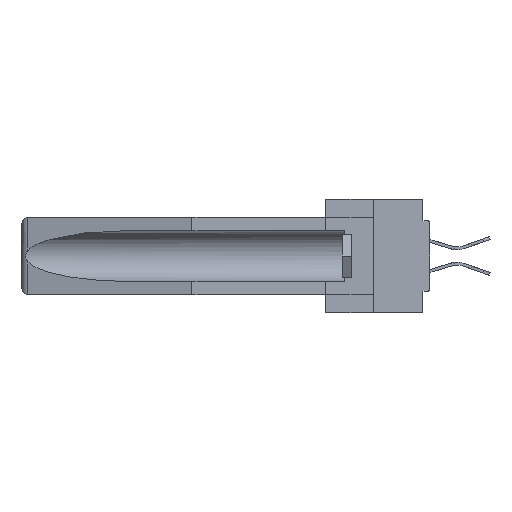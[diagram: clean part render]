
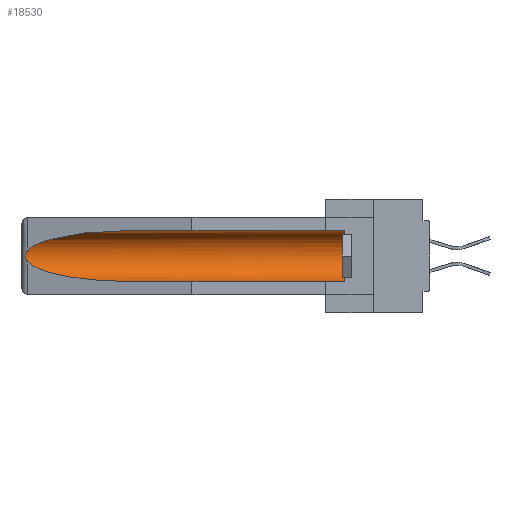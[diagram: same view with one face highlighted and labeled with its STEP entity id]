
A CAD part, left-side view. The second image highlights one B-rep face of the part: STEP entity #18530.
In plain terms, the highlighted cylindrical face has radius 2.857 mm (diameter 5.715 mm), a partial arc.
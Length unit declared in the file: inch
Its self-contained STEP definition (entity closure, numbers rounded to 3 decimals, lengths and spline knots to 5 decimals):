
#882 = AXIS2_PLACEMENT_3D ( 'NONE', #37598, #18203, #40894 ) ;
#1611 = CARTESIAN_POINT ( 'NONE',  ( 0.26537, 1.52718, -0.14972 ) ) ;
#3280 = CARTESIAN_POINT ( 'NONE',  ( 0.26597, 1.5296, -0.19026 ) ) ;
#3557 = CARTESIAN_POINT ( 'NONE',  ( 0.26537, 1.52718, -0.19328 ) ) ;
#3558 = VECTOR ( 'NONE', #12889, 39.37008 ) ;
#3922 = ORIENTED_EDGE ( 'NONE', *, *, #5199, .T. ) ;
#5050 = CARTESIAN_POINT ( 'NONE',  ( 0.155, -0.30754, -0.1715 ) ) ;
#5131 = ORIENTED_EDGE ( 'NONE', *, *, #38512, .T. ) ;
#5199 = EDGE_CURVE ( 'NONE', #19929, #33676, #34286, .T. ) ;
#6476 = CARTESIAN_POINT ( 'NONE',  ( 0.26597, 1.52961, -0.15275 ) ) ;
#9622 = EDGE_CURVE ( 'NONE', #16910, #29079, #25390, .T. ) ;
#9692 = CARTESIAN_POINT ( 'NONE',  ( 0.2673, 1.53269, -0.17917 ) ) ;
#10557 = EDGE_LOOP ( 'NONE', ( #22470, #5131, #3922, #35217, #26664, #25958 ) ) ;
#10657 = EDGE_CURVE ( 'NONE', #10664, #16910, #38029, .T. ) ;
#10664 = VERTEX_POINT ( 'NONE', #16553 ) ;
#11248 = VECTOR ( 'NONE', #35935, 39.37008 ) ;
#12256 = CARTESIAN_POINT ( 'NONE',  ( 0.25451, 1.48313, -0.24835 ) ) ;
#12609 = CARTESIAN_POINT ( 'NONE',  ( 0.2675, 1.53308, -0.16763 ) ) ;
#12748 = CARTESIAN_POINT ( 'NONE',  ( 0.155, -0.30754, -0.284 ) ) ;
#12889 = DIRECTION ( 'NONE',  ( 0., 1., 0. ) ) ;
#14210 = FACE_OUTER_BOUND ( 'NONE', #10557, .T. ) ;
#14325 = CARTESIAN_POINT ( 'NONE',  ( 0.26537, 1.52718, -0.19328 ) ) ;
#16044 = CARTESIAN_POINT ( 'NONE',  ( 0.155, 1.07973, -0.284 ) ) ;
#16129 = CARTESIAN_POINT ( 'NONE',  ( 0.2673, 1.5327, -0.16383 ) ) ;
#16184 = CARTESIAN_POINT ( 'NONE',  ( 0.21114, 1.30732, -0.284 ) ) ;
#16553 = CARTESIAN_POINT ( 'NONE',  ( 0.155, 0.126, -0.059 ) ) ;
#16910 = VERTEX_POINT ( 'NONE', #19436 ) ;
#18069 = DIRECTION ( 'NONE',  ( 0., 1., 0. ) ) ;
#18203 = DIRECTION ( 'NONE',  ( 0., -1., 0. ) ) ;
#18367 = CARTESIAN_POINT ( 'NONE',  ( 0.155, 1.07973, -0.284 ) ) ;
#18530 = ADVANCED_FACE ( 'NONE', ( #14210 ), #31381, .F. ) ;
#18571 = EDGE_CURVE ( 'NONE', #36575, #10664, #24782, .T. ) ;
#18821 = CARTESIAN_POINT ( 'NONE',  ( 0.26537, 1.52718, -0.19328 ) ) ;
#19436 = CARTESIAN_POINT ( 'NONE',  ( 0.155, 1.07973, -0.059 ) ) ;
#19929 = VERTEX_POINT ( 'NONE', #14325 ) ;
#21216 = CARTESIAN_POINT ( 'NONE',  ( 0.25451, 1.48313, -0.09465 ) ) ;
#21594 = LINE ( 'NONE', #12748, #3558 ) ;
#22470 = ORIENTED_EDGE ( 'NONE', *, *, #9622, .T. ) ;
#22479 = CARTESIAN_POINT ( 'NONE',  ( 0.26655, 1.53094, -0.18657 ) ) ;
#22613 = CARTESIAN_POINT ( 'NONE',  ( 0.155, -0.30754, -0.059 ) ) ;
#23965 = CARTESIAN_POINT ( 'NONE',  ( 0.155, 1.07973, -0.059 ) ) ;
#24782 = CIRCLE ( 'NONE', #882, 0.1125 ) ;
#25390 =( BOUNDED_CURVE ( )  B_SPLINE_CURVE ( 3, ( #23965, #30434, #21216, #36985 ),
 .UNSPECIFIED., .F., .F. ) 
 B_SPLINE_CURVE_WITH_KNOTS ( ( 4, 4 ),
 ( 4.71239, 6.08839 ),
 .UNSPECIFIED. ) 
 CURVE ( )  GEOMETRIC_REPRESENTATION_ITEM ( )  RATIONAL_B_SPLINE_CURVE ( ( 1., 0.848, 0.848, 1. ) ) 
 REPRESENTATION_ITEM ( '' )  );
#25958 = ORIENTED_EDGE ( 'NONE', *, *, #10657, .T. ) ;
#26664 = ORIENTED_EDGE ( 'NONE', *, *, #18571, .T. ) ;
#29079 = VERTEX_POINT ( 'NONE', #1611 ) ;
#29086 = CARTESIAN_POINT ( 'NONE',  ( 0.2675, 1.53308, -0.17534 ) ) ;
#29150 = CARTESIAN_POINT ( 'NONE',  ( 0.155, 0.126, -0.284 ) ) ;
#30434 = CARTESIAN_POINT ( 'NONE',  ( 0.21114, 1.30732, -0.059 ) ) ;
#31381 = CYLINDRICAL_SURFACE ( 'NONE', #35075, 0.1125 ) ;
#33676 = VERTEX_POINT ( 'NONE', #16044 ) ;
#34286 =( BOUNDED_CURVE ( )  B_SPLINE_CURVE ( 3, ( #18821, #12256, #16184, #18367 ),
 .UNSPECIFIED., .F., .F. ) 
 B_SPLINE_CURVE_WITH_KNOTS ( ( 4, 4 ),
 ( 0.1948, 1.5708 ),
 .UNSPECIFIED. ) 
 CURVE ( )  GEOMETRIC_REPRESENTATION_ITEM ( )  RATIONAL_B_SPLINE_CURVE ( ( 1., 0.848, 0.848, 1. ) ) 
 REPRESENTATION_ITEM ( '' )  );
#35075 = AXIS2_PLACEMENT_3D ( 'NONE', #5050, #18069, #41032 ) ;
#35217 = ORIENTED_EDGE ( 'NONE', *, *, #38483, .F. ) ;
#35935 = DIRECTION ( 'NONE',  ( 0., 1., 0. ) ) ;
#36575 = VERTEX_POINT ( 'NONE', #29150 ) ;
#36985 = CARTESIAN_POINT ( 'NONE',  ( 0.26537, 1.52718, -0.14972 ) ) ;
#37598 = CARTESIAN_POINT ( 'NONE',  ( 0.155, 0.126, -0.1715 ) ) ;
#38029 = LINE ( 'NONE', #22613, #11248 ) ;
#38483 = EDGE_CURVE ( 'NONE', #36575, #33676, #21594, .T. ) ;
#38503 = CARTESIAN_POINT ( 'NONE',  ( 0.26537, 1.52718, -0.14972 ) ) ;
#38512 = EDGE_CURVE ( 'NONE', #29079, #19929, #38708, .T. ) ;
#38638 = CARTESIAN_POINT ( 'NONE',  ( 0.26654, 1.53092, -0.15636 ) ) ;
#38708 = B_SPLINE_CURVE_WITH_KNOTS ( 'NONE', 3,
 ( #38503, #6476, #38638, #16129, #12609, #29086, #9692, #22479, #3280, #3557 ),
 .UNSPECIFIED., .F., .F.,
 ( 4, 2, 2, 2, 4 ),
 ( 0., 0.00029, 0.00058, 0.00087, 0.00117 ),
 .UNSPECIFIED. ) ;
#40894 = DIRECTION ( 'NONE',  ( 0., 0., 1. ) ) ;
#41032 = DIRECTION ( 'NONE',  ( 0., 0., 1. ) ) ;
